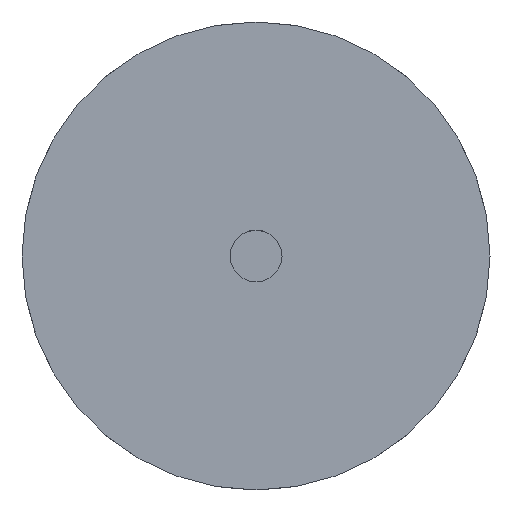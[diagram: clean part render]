
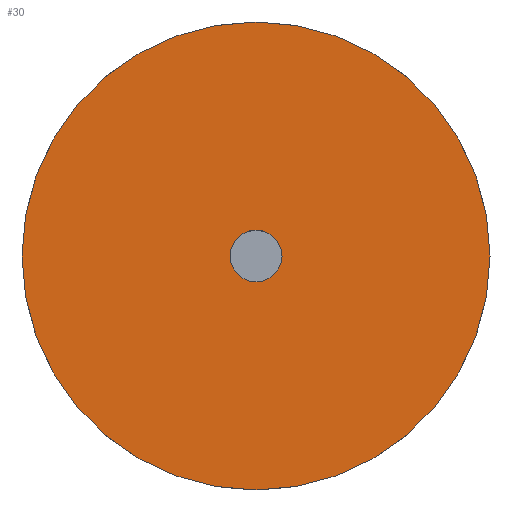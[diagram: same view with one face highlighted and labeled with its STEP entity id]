
A CAD part, top view. The second image highlights one B-rep face of the part: STEP entity #30.
In plain terms, the highlighted planar face has unit normal (0, 0, 1).
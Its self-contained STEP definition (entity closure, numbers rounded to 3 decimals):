
#5 = AXIS2_PLACEMENT_3D ( 'NONE', #202, #69, #22 ) ;
#10 = CIRCLE ( 'NONE', #5, 4.5 ) ;
#12 = CIRCLE ( 'NONE', #138, 4.5 ) ;
#22 = DIRECTION ( 'NONE',  ( 1., 0., 0. ) ) ;
#25 = FACE_OUTER_BOUND ( 'NONE', #85, .T. ) ;
#30 = ADVANCED_FACE ( 'NONE', ( #136, #25 ), #139, .F. ) ;
#44 = CARTESIAN_POINT ( 'NONE',  ( 0., 0., 0. ) ) ;
#47 = ORIENTED_EDGE ( 'NONE', *, *, #241, .T. ) ;
#69 = DIRECTION ( 'NONE',  ( 0., 0., 1. ) ) ;
#85 = EDGE_LOOP ( 'NONE', ( #272, #47 ) ) ;
#89 = AXIS2_PLACEMENT_3D ( 'NONE', #223, #219, #213 ) ;
#93 = VERTEX_POINT ( 'NONE', #253 ) ;
#103 = EDGE_LOOP ( 'NONE', ( #232, #308 ) ) ;
#121 = VERTEX_POINT ( 'NONE', #187 ) ;
#126 = EDGE_CURVE ( 'NONE', #134, #93, #316, .T. ) ;
#128 = CARTESIAN_POINT ( 'NONE',  ( 0., 0., 0. ) ) ;
#134 = VERTEX_POINT ( 'NONE', #247 ) ;
#136 = FACE_BOUND ( 'NONE', #103, .T. ) ;
#137 = DIRECTION ( 'NONE',  ( -1., 0., 0. ) ) ;
#138 = AXIS2_PLACEMENT_3D ( 'NONE', #44, #296, #317 ) ;
#139 = PLANE ( 'NONE',  #217 ) ;
#153 = EDGE_CURVE ( 'NONE', #236, #121, #10, .T. ) ;
#170 = CARTESIAN_POINT ( 'NONE',  ( 0., 0., 0. ) ) ;
#181 = DIRECTION ( 'NONE',  ( 0., 0., 1. ) ) ;
#187 = CARTESIAN_POINT ( 'NONE',  ( -4.5, 0., 0. ) ) ;
#198 = AXIS2_PLACEMENT_3D ( 'NONE', #128, #181, #201 ) ;
#201 = DIRECTION ( 'NONE',  ( 1., 0., 0. ) ) ;
#202 = CARTESIAN_POINT ( 'NONE',  ( 0., 0., 0. ) ) ;
#213 = DIRECTION ( 'NONE',  ( 1., 0., 0. ) ) ;
#217 = AXIS2_PLACEMENT_3D ( 'NONE', #170, #318, #137 ) ;
#219 = DIRECTION ( 'NONE',  ( 0., 0., 1. ) ) ;
#223 = CARTESIAN_POINT ( 'NONE',  ( 0., 0., 0. ) ) ;
#232 = ORIENTED_EDGE ( 'NONE', *, *, #256, .F. ) ;
#236 = VERTEX_POINT ( 'NONE', #281 ) ;
#241 = EDGE_CURVE ( 'NONE', #121, #236, #12, .T. ) ;
#247 = CARTESIAN_POINT ( 'NONE',  ( -0.5, 0., 0. ) ) ;
#253 = CARTESIAN_POINT ( 'NONE',  ( 0.5, 0., 0. ) ) ;
#256 = EDGE_CURVE ( 'NONE', #93, #134, #307, .T. ) ;
#272 = ORIENTED_EDGE ( 'NONE', *, *, #153, .T. ) ;
#281 = CARTESIAN_POINT ( 'NONE',  ( 4.5, 0., 0. ) ) ;
#296 = DIRECTION ( 'NONE',  ( 0., 0., 1. ) ) ;
#307 = CIRCLE ( 'NONE', #89, 0.5 ) ;
#308 = ORIENTED_EDGE ( 'NONE', *, *, #126, .F. ) ;
#316 = CIRCLE ( 'NONE', #198, 0.5 ) ;
#317 = DIRECTION ( 'NONE',  ( 1., 0., 0. ) ) ;
#318 = DIRECTION ( 'NONE',  ( 0., 0., -1. ) ) ;
